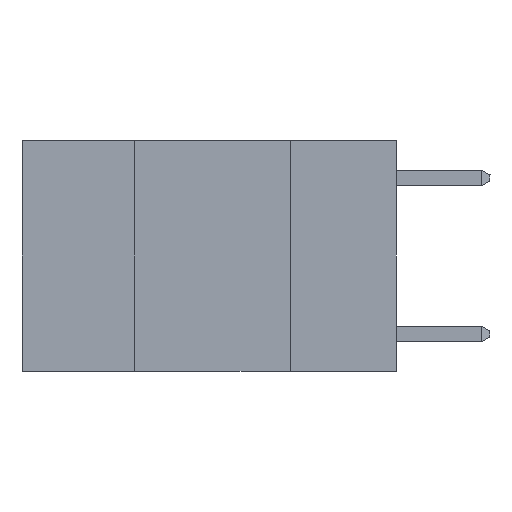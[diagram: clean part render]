
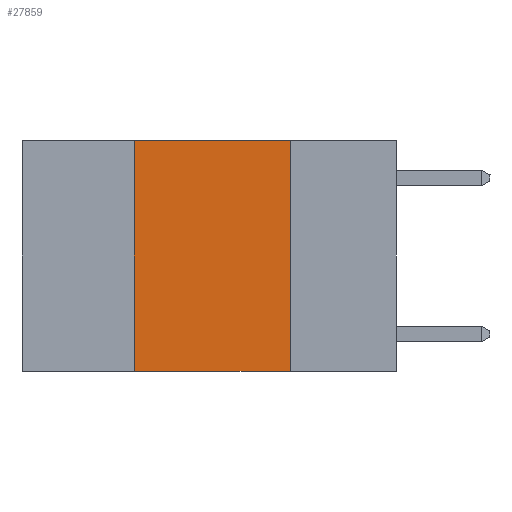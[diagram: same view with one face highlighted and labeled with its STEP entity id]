
A CAD part, left-side view. The second image highlights one B-rep face of the part: STEP entity #27859.
In plain terms, the highlighted planar face has unit normal (-1, 0, 0).
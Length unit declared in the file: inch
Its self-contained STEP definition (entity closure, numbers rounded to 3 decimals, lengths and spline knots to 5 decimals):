
#1653 = EDGE_CURVE ( 'NONE', #11858, #6071, #10343, .T. ) ;
#2162 = LINE ( 'NONE', #26220, #24520 ) ;
#2283 = EDGE_CURVE ( 'NONE', #6071, #10154, #5383, .T. ) ;
#2396 = LINE ( 'NONE', #12435, #10624 ) ;
#2553 = ORIENTED_EDGE ( 'NONE', *, *, #1653, .F. ) ;
#2562 = CARTESIAN_POINT ( 'NONE',  ( 0., 0.17, 0. ) ) ;
#4028 = CARTESIAN_POINT ( 'NONE',  ( 0., 0.42, 0. ) ) ;
#5383 = LINE ( 'NONE', #7496, #16633 ) ;
#5887 = FACE_OUTER_BOUND ( 'NONE', #23036, .T. ) ;
#6071 = VERTEX_POINT ( 'NONE', #4028 ) ;
#6208 = CARTESIAN_POINT ( 'NONE',  ( 0., 0.6, 0. ) ) ;
#7496 = CARTESIAN_POINT ( 'NONE',  ( 0., 0.6, 0. ) ) ;
#9036 = CARTESIAN_POINT ( 'NONE',  ( 0., 0.42, -0.37 ) ) ;
#10123 = EDGE_CURVE ( 'NONE', #10154, #14899, #2396, .T. ) ;
#10154 = VERTEX_POINT ( 'NONE', #2562 ) ;
#10343 = LINE ( 'NONE', #20230, #13688 ) ;
#10624 = VECTOR ( 'NONE', #12268, 39.37008 ) ;
#11858 = VERTEX_POINT ( 'NONE', #9036 ) ;
#12268 = DIRECTION ( 'NONE',  ( 0., 0., -1. ) ) ;
#12435 = CARTESIAN_POINT ( 'NONE',  ( 0., 0.17, 0. ) ) ;
#13688 = VECTOR ( 'NONE', #30027, 39.37008 ) ;
#14899 = VERTEX_POINT ( 'NONE', #18519 ) ;
#14956 = DIRECTION ( 'NONE',  ( 0., -1., 0. ) ) ;
#16633 = VECTOR ( 'NONE', #14956, 39.37008 ) ;
#18519 = CARTESIAN_POINT ( 'NONE',  ( 0., 0.17, -0.37 ) ) ;
#18936 = ORIENTED_EDGE ( 'NONE', *, *, #2283, .F. ) ;
#20230 = CARTESIAN_POINT ( 'NONE',  ( 0., 0.42, 0. ) ) ;
#21223 = EDGE_CURVE ( 'NONE', #11858, #14899, #2162, .T. ) ;
#21240 = PLANE ( 'NONE',  #28348 ) ;
#21569 = DIRECTION ( 'NONE',  ( 0., -1., 0. ) ) ;
#21938 = ORIENTED_EDGE ( 'NONE', *, *, #21223, .T. ) ;
#23036 = EDGE_LOOP ( 'NONE', ( #27828, #18936, #2553, #21938 ) ) ;
#23185 = DIRECTION ( 'NONE',  ( 1., 0., 0. ) ) ;
#24520 = VECTOR ( 'NONE', #21569, 39.37008 ) ;
#26220 = CARTESIAN_POINT ( 'NONE',  ( 0., 0.6, -0.37 ) ) ;
#27828 = ORIENTED_EDGE ( 'NONE', *, *, #10123, .F. ) ;
#27859 = ADVANCED_FACE ( 'NONE', ( #5887 ), #21240, .F. ) ;
#28348 = AXIS2_PLACEMENT_3D ( 'NONE', #6208, #23185, #31067 ) ;
#30027 = DIRECTION ( 'NONE',  ( 0., 0., 1. ) ) ;
#31067 = DIRECTION ( 'NONE',  ( 0., 0., -1. ) ) ;
